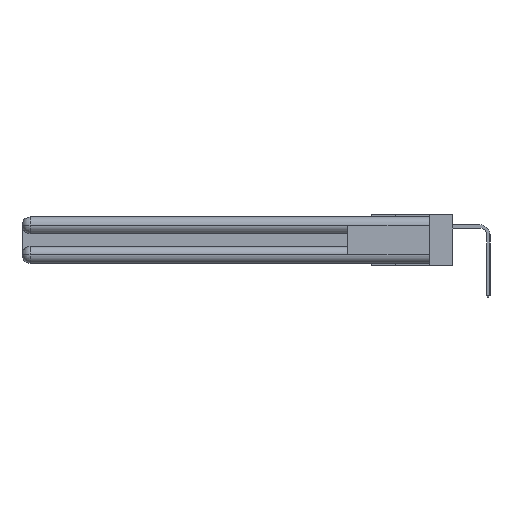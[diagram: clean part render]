
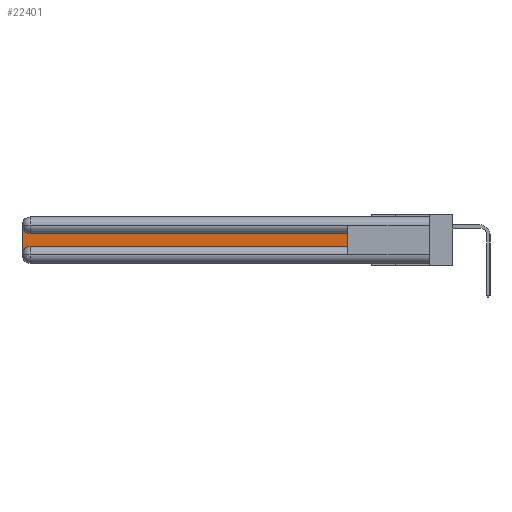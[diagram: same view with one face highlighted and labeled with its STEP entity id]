
A CAD part, left-side view. The second image highlights one B-rep face of the part: STEP entity #22401.
In plain terms, the highlighted planar face has unit normal (-1, 0, 0).
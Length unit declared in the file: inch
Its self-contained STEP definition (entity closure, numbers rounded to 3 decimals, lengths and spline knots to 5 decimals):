
#551 = CARTESIAN_POINT ( 'NONE',  ( 0.075, 2.94, -0.2775 ) ) ;
#1114 = DIRECTION ( 'NONE',  ( 0., -1., 0. ) ) ;
#1895 = CARTESIAN_POINT ( 'NONE',  ( 0.075, 3., -0.2775 ) ) ;
#2494 = LINE ( 'NONE', #14305, #7833 ) ;
#3264 = VECTOR ( 'NONE', #12142, 39.37008 ) ;
#3544 = VERTEX_POINT ( 'NONE', #18332 ) ;
#5147 = EDGE_CURVE ( 'NONE', #9949, #9740, #13408, .T. ) ;
#6244 = LINE ( 'NONE', #11539, #19880 ) ;
#6898 = ORIENTED_EDGE ( 'NONE', *, *, #24423, .T. ) ;
#7630 = CARTESIAN_POINT ( 'NONE',  ( 0.075, 0.6, -0.2175 ) ) ;
#7833 = VECTOR ( 'NONE', #1114, 39.37008 ) ;
#8648 = ORIENTED_EDGE ( 'NONE', *, *, #13928, .T. ) ;
#9740 = VERTEX_POINT ( 'NONE', #18648 ) ;
#9949 = VERTEX_POINT ( 'NONE', #1895 ) ;
#10044 = VECTOR ( 'NONE', #24110, 39.37008 ) ;
#11156 = CARTESIAN_POINT ( 'NONE',  ( 0.075, 0.6, -0.2175 ) ) ;
#11539 = CARTESIAN_POINT ( 'NONE',  ( 0.075, 0.6, -0.1225 ) ) ;
#12142 = DIRECTION ( 'NONE',  ( 0., 0., 1. ) ) ;
#13280 = ORIENTED_EDGE ( 'NONE', *, *, #26673, .T. ) ;
#13355 = VERTEX_POINT ( 'NONE', #25215 ) ;
#13408 = CIRCLE ( 'NONE', #21754, 0.06 ) ;
#13928 = EDGE_CURVE ( 'NONE', #13355, #9949, #17749, .T. ) ;
#14089 = PLANE ( 'NONE',  #22228 ) ;
#14230 = DIRECTION ( 'NONE',  ( 0., 0., -1. ) ) ;
#14305 = CARTESIAN_POINT ( 'NONE',  ( 0.075, 0.6, -0.2175 ) ) ;
#14599 = EDGE_CURVE ( 'NONE', #9740, #16177, #2494, .T. ) ;
#14607 = VERTEX_POINT ( 'NONE', #26141 ) ;
#14967 = CIRCLE ( 'NONE', #28204, 0.06 ) ;
#15217 = CARTESIAN_POINT ( 'NONE',  ( 0.075, 3., -0.2175 ) ) ;
#16177 = VERTEX_POINT ( 'NONE', #11156 ) ;
#16307 = DIRECTION ( 'NONE',  ( 1., 0., 0. ) ) ;
#17749 = LINE ( 'NONE', #15217, #10044 ) ;
#18332 = CARTESIAN_POINT ( 'NONE',  ( 0.075, 2.94, -0.1225 ) ) ;
#18469 = DIRECTION ( 'NONE',  ( 0., 1., 0. ) ) ;
#18648 = CARTESIAN_POINT ( 'NONE',  ( 0.075, 2.94, -0.2175 ) ) ;
#19341 = EDGE_CURVE ( 'NONE', #3544, #13355, #14967, .T. ) ;
#19880 = VECTOR ( 'NONE', #18469, 39.37008 ) ;
#20513 = CARTESIAN_POINT ( 'NONE',  ( 0.075, 3., -0.1225 ) ) ;
#20871 = LINE ( 'NONE', #7630, #3264 ) ;
#21754 = AXIS2_PLACEMENT_3D ( 'NONE', #551, #27627, #14230 ) ;
#22228 = AXIS2_PLACEMENT_3D ( 'NONE', #20513, #22868, #27396 ) ;
#22401 = ADVANCED_FACE ( 'NONE', ( #26969 ), #14089, .F. ) ;
#22868 = DIRECTION ( 'NONE',  ( 1., 0., 0. ) ) ;
#23359 = ORIENTED_EDGE ( 'NONE', *, *, #19341, .T. ) ;
#23791 = ORIENTED_EDGE ( 'NONE', *, *, #5147, .T. ) ;
#24110 = DIRECTION ( 'NONE',  ( 0., 0., -1. ) ) ;
#24423 = EDGE_CURVE ( 'NONE', #16177, #14607, #20871, .T. ) ;
#24676 = ORIENTED_EDGE ( 'NONE', *, *, #14599, .T. ) ;
#25035 = DIRECTION ( 'NONE',  ( 0., 0., -1. ) ) ;
#25215 = CARTESIAN_POINT ( 'NONE',  ( 0.075, 3., -0.0625 ) ) ;
#26141 = CARTESIAN_POINT ( 'NONE',  ( 0.075, 0.6, -0.1225 ) ) ;
#26673 = EDGE_CURVE ( 'NONE', #14607, #3544, #6244, .T. ) ;
#26912 = EDGE_LOOP ( 'NONE', ( #13280, #23359, #8648, #23791, #24676, #6898 ) ) ;
#26969 = FACE_OUTER_BOUND ( 'NONE', #26912, .T. ) ;
#27396 = DIRECTION ( 'NONE',  ( 0., 0., -1. ) ) ;
#27571 = CARTESIAN_POINT ( 'NONE',  ( 0.075, 2.94, -0.0625 ) ) ;
#27627 = DIRECTION ( 'NONE',  ( 1., 0., 0. ) ) ;
#28204 = AXIS2_PLACEMENT_3D ( 'NONE', #27571, #16307, #25035 ) ;
